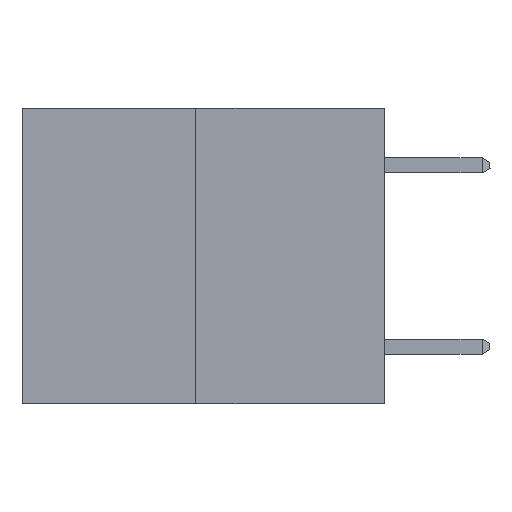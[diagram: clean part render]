
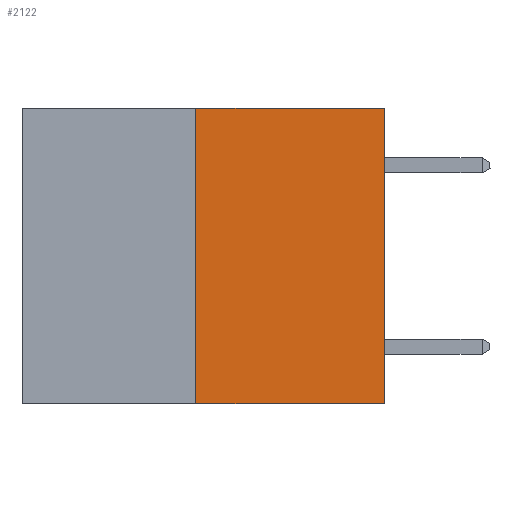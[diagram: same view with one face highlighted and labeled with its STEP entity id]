
A CAD part, left-side view. The second image highlights one B-rep face of the part: STEP entity #2122.
In plain terms, the highlighted planar face has unit normal (-1, 0, 0).
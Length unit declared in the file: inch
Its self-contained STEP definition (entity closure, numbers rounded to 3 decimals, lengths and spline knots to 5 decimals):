
#368 = ORIENTED_EDGE ( 'NONE', *, *, #8304, .T. ) ;
#378 = PLANE ( 'NONE',  #16011 ) ;
#804 = VERTEX_POINT ( 'NONE', #6339 ) ;
#1599 = VECTOR ( 'NONE', #16260, 39.37008 ) ;
#1909 = CARTESIAN_POINT ( 'NONE',  ( 0., 0.6, -0.49 ) ) ;
#2122 = ADVANCED_FACE ( 'NONE', ( #19911 ), #378, .F. ) ;
#2738 = VECTOR ( 'NONE', #6609, 39.37008 ) ;
#4454 = LINE ( 'NONE', #1909, #1599 ) ;
#4730 = DIRECTION ( 'NONE',  ( 0., 0., -1. ) ) ;
#5177 = EDGE_CURVE ( 'NONE', #8156, #15756, #13119, .T. ) ;
#5185 = ORIENTED_EDGE ( 'NONE', *, *, #7460, .F. ) ;
#6339 = CARTESIAN_POINT ( 'NONE',  ( 0., 0., -0.49 ) ) ;
#6411 = CARTESIAN_POINT ( 'NONE',  ( 0., 0., 0. ) ) ;
#6609 = DIRECTION ( 'NONE',  ( 0., -1., 0. ) ) ;
#7460 = EDGE_CURVE ( 'NONE', #22120, #8156, #16775, .T. ) ;
#7681 = CARTESIAN_POINT ( 'NONE',  ( 0., 0., 0. ) ) ;
#8156 = VERTEX_POINT ( 'NONE', #19668 ) ;
#8304 = EDGE_CURVE ( 'NONE', #22120, #804, #4454, .T. ) ;
#8952 = EDGE_CURVE ( 'NONE', #804, #15756, #12023, .T. ) ;
#10597 = CARTESIAN_POINT ( 'NONE',  ( 0., 0.6, 0. ) ) ;
#10792 = ORIENTED_EDGE ( 'NONE', *, *, #8952, .T. ) ;
#12023 = LINE ( 'NONE', #6411, #21584 ) ;
#13119 = LINE ( 'NONE', #10597, #2738 ) ;
#14140 = DIRECTION ( 'NONE',  ( 0., 0., 1. ) ) ;
#14616 = DIRECTION ( 'NONE',  ( 0., 0., 1. ) ) ;
#15756 = VERTEX_POINT ( 'NONE', #7681 ) ;
#16011 = AXIS2_PLACEMENT_3D ( 'NONE', #24526, #18659, #4730 ) ;
#16260 = DIRECTION ( 'NONE',  ( 0., -1., 0. ) ) ;
#16329 = CARTESIAN_POINT ( 'NONE',  ( 0., 0.312, -0.49 ) ) ;
#16775 = LINE ( 'NONE', #16329, #19632 ) ;
#18659 = DIRECTION ( 'NONE',  ( 1., 0., 0. ) ) ;
#19225 = EDGE_LOOP ( 'NONE', ( #5185, #368, #10792, #19744 ) ) ;
#19632 = VECTOR ( 'NONE', #14140, 39.37008 ) ;
#19668 = CARTESIAN_POINT ( 'NONE',  ( 0., 0.312, 0. ) ) ;
#19744 = ORIENTED_EDGE ( 'NONE', *, *, #5177, .F. ) ;
#19911 = FACE_OUTER_BOUND ( 'NONE', #19225, .T. ) ;
#21142 = CARTESIAN_POINT ( 'NONE',  ( 0., 0.312, -0.49 ) ) ;
#21584 = VECTOR ( 'NONE', #14616, 39.37008 ) ;
#22120 = VERTEX_POINT ( 'NONE', #21142 ) ;
#24526 = CARTESIAN_POINT ( 'NONE',  ( 0., 0.6, 0. ) ) ;
